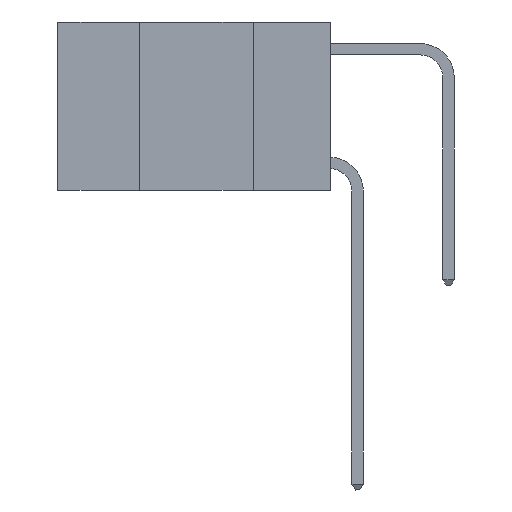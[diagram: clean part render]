
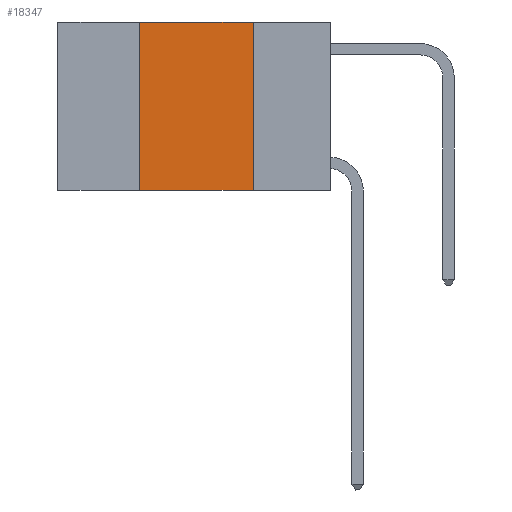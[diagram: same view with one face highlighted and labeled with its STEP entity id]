
A CAD part, left-side view. The second image highlights one B-rep face of the part: STEP entity #18347.
In plain terms, the highlighted planar face has unit normal (-1, 0, 0).
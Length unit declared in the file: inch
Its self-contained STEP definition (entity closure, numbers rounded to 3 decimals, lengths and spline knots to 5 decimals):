
#2358 = VECTOR ( 'NONE', #6266, 39.37008 ) ;
#3108 = VERTEX_POINT ( 'NONE', #6332 ) ;
#3582 = ORIENTED_EDGE ( 'NONE', *, *, #20681, .T. ) ;
#4355 = LINE ( 'NONE', #14616, #4655 ) ;
#4464 = ORIENTED_EDGE ( 'NONE', *, *, #17952, .F. ) ;
#4655 = VECTOR ( 'NONE', #18257, 39.37008 ) ;
#5018 = VECTOR ( 'NONE', #11244, 39.37008 ) ;
#5050 = CARTESIAN_POINT ( 'NONE',  ( 0., 0.42, 0. ) ) ;
#5740 = AXIS2_PLACEMENT_3D ( 'NONE', #9188, #19308, #17724 ) ;
#5754 = VECTOR ( 'NONE', #19719, 39.37008 ) ;
#6156 = LINE ( 'NONE', #9514, #2358 ) ;
#6266 = DIRECTION ( 'NONE',  ( 0., 0., 1. ) ) ;
#6332 = CARTESIAN_POINT ( 'NONE',  ( 0., 0.17, -0.37 ) ) ;
#7796 = LINE ( 'NONE', #14607, #5754 ) ;
#9188 = CARTESIAN_POINT ( 'NONE',  ( 0., 0.6, 0. ) ) ;
#9514 = CARTESIAN_POINT ( 'NONE',  ( 0., 0.42, 0. ) ) ;
#9679 = CARTESIAN_POINT ( 'NONE',  ( 0., 0.42, -0.37 ) ) ;
#10253 = VERTEX_POINT ( 'NONE', #5050 ) ;
#10910 = LINE ( 'NONE', #14468, #5018 ) ;
#11244 = DIRECTION ( 'NONE',  ( 0., -1., 0. ) ) ;
#11712 = EDGE_CURVE ( 'NONE', #13886, #10253, #6156, .T. ) ;
#13886 = VERTEX_POINT ( 'NONE', #9679 ) ;
#14185 = PLANE ( 'NONE',  #5740 ) ;
#14289 = FACE_OUTER_BOUND ( 'NONE', #15393, .T. ) ;
#14468 = CARTESIAN_POINT ( 'NONE',  ( 0., 0.6, -0.37 ) ) ;
#14607 = CARTESIAN_POINT ( 'NONE',  ( 0., 0.17, 0. ) ) ;
#14616 = CARTESIAN_POINT ( 'NONE',  ( 0., 0.6, 0. ) ) ;
#15393 = EDGE_LOOP ( 'NONE', ( #21661, #4464, #20783, #3582 ) ) ;
#16602 = CARTESIAN_POINT ( 'NONE',  ( 0., 0.17, 0. ) ) ;
#17724 = DIRECTION ( 'NONE',  ( 0., 0., -1. ) ) ;
#17952 = EDGE_CURVE ( 'NONE', #10253, #20465, #4355, .T. ) ;
#18257 = DIRECTION ( 'NONE',  ( 0., -1., 0. ) ) ;
#18347 = ADVANCED_FACE ( 'NONE', ( #14289 ), #14185, .F. ) ;
#19014 = EDGE_CURVE ( 'NONE', #20465, #3108, #7796, .T. ) ;
#19308 = DIRECTION ( 'NONE',  ( 1., 0., 0. ) ) ;
#19719 = DIRECTION ( 'NONE',  ( 0., 0., -1. ) ) ;
#20465 = VERTEX_POINT ( 'NONE', #16602 ) ;
#20681 = EDGE_CURVE ( 'NONE', #13886, #3108, #10910, .T. ) ;
#20783 = ORIENTED_EDGE ( 'NONE', *, *, #11712, .F. ) ;
#21661 = ORIENTED_EDGE ( 'NONE', *, *, #19014, .F. ) ;
